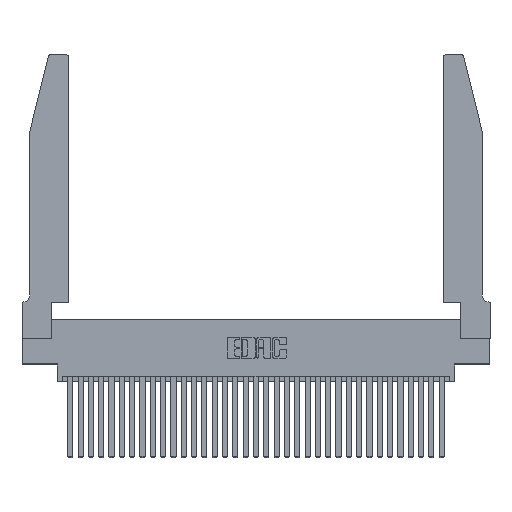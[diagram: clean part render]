
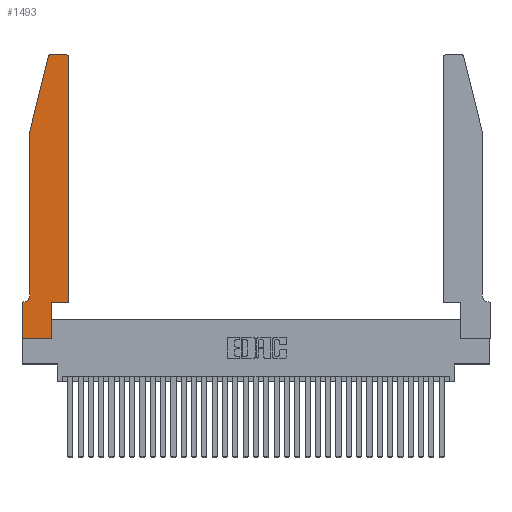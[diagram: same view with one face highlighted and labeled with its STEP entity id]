
A CAD part, top view. The second image highlights one B-rep face of the part: STEP entity #1493.
In plain terms, the highlighted planar face has unit normal (0, 0, 1).
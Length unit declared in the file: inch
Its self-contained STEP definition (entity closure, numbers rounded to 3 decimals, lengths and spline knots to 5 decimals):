
#58 = CARTESIAN_POINT ( 'NONE',  ( 0.284, 2.72, 0.37 ) ) ;
#142 = LINE ( 'NONE', #5960, #14579 ) ;
#613 = ORIENTED_EDGE ( 'NONE', *, *, #21931, .T. ) ;
#890 = DIRECTION ( 'NONE',  ( -1., 0., 0. ) ) ;
#907 = CARTESIAN_POINT ( 'NONE',  ( 0.0755, 2., 0.37 ) ) ;
#1493 = ADVANCED_FACE ( 'NONE', ( #13940 ), #15203, .T. ) ;
#1640 = VERTEX_POINT ( 'NONE', #9543 ) ;
#1760 = VECTOR ( 'NONE', #22726, 39.37008 ) ;
#1867 = VECTOR ( 'NONE', #25450, 39.37008 ) ;
#2013 = CIRCLE ( 'NONE', #11670, 0.03 ) ;
#2410 = VECTOR ( 'NONE', #11007, 39.37008 ) ;
#2797 = ORIENTED_EDGE ( 'NONE', *, *, #31492, .T. ) ;
#2894 = DIRECTION ( 'NONE',  ( 1., 0., 0. ) ) ;
#2965 = VECTOR ( 'NONE', #29072, 39.37008 ) ;
#4158 = LINE ( 'NONE', #26662, #2410 ) ;
#4244 = CARTESIAN_POINT ( 'NONE',  ( 0., 0., 0.37 ) ) ;
#5217 = EDGE_CURVE ( 'NONE', #7828, #17692, #23101, .T. ) ;
#5246 = VERTEX_POINT ( 'NONE', #30974 ) ;
#5944 = DIRECTION ( 'NONE',  ( 0., 1., 0. ) ) ;
#5960 = CARTESIAN_POINT ( 'NONE',  ( 0.0755, 2., 0.37 ) ) ;
#6598 = CARTESIAN_POINT ( 'NONE',  ( 0.25487, 2.72718, 0.37 ) ) ;
#6966 = CARTESIAN_POINT ( 'NONE',  ( 0.2605, 2.75, 0.37 ) ) ;
#7046 = DIRECTION ( 'NONE',  ( 0., 0., 1. ) ) ;
#7828 = VERTEX_POINT ( 'NONE', #10424 ) ;
#7961 = ORIENTED_EDGE ( 'NONE', *, *, #5217, .T. ) ;
#8370 = ORIENTED_EDGE ( 'NONE', *, *, #20316, .T. ) ;
#8818 = ORIENTED_EDGE ( 'NONE', *, *, #14589, .T. ) ;
#9064 = CARTESIAN_POINT ( 'NONE',  ( 0.0055, 0.35, 0.37 ) ) ;
#9543 = CARTESIAN_POINT ( 'NONE',  ( 0.0755, 0.42, 0.37 ) ) ;
#10069 = ORIENTED_EDGE ( 'NONE', *, *, #23558, .T. ) ;
#10424 = CARTESIAN_POINT ( 'NONE',  ( 0.4505, 0.35, 0.37 ) ) ;
#10915 = EDGE_CURVE ( 'NONE', #32493, #16985, #23509, .T. ) ;
#11007 = DIRECTION ( 'NONE',  ( -1., 0., 0. ) ) ;
#11014 = VERTEX_POINT ( 'NONE', #20634 ) ;
#11587 = CARTESIAN_POINT ( 'NONE',  ( 0., 0.35, 0.37 ) ) ;
#11670 = AXIS2_PLACEMENT_3D ( 'NONE', #22809, #7046, #25445 ) ;
#12025 = EDGE_CURVE ( 'NONE', #17823, #5246, #16896, .T. ) ;
#13385 = CARTESIAN_POINT ( 'NONE',  ( 0.4505, 0.35, 0.37 ) ) ;
#13393 = ORIENTED_EDGE ( 'NONE', *, *, #20196, .T. ) ;
#13940 = FACE_OUTER_BOUND ( 'NONE', #31649, .T. ) ;
#14579 = VECTOR ( 'NONE', #24386, 39.37008 ) ;
#14589 = EDGE_CURVE ( 'NONE', #17692, #17823, #2013, .T. ) ;
#14602 = ORIENTED_EDGE ( 'NONE', *, *, #12025, .T. ) ;
#14742 = DIRECTION ( 'NONE',  ( 1., 0., 0. ) ) ;
#14877 = CARTESIAN_POINT ( 'NONE',  ( 0.4505, 2.72, 0.37 ) ) ;
#14972 = DIRECTION ( 'NONE',  ( 0., 0., 1. ) ) ;
#15203 = PLANE ( 'NONE',  #16921 ) ;
#15237 = VECTOR ( 'NONE', #19773, 39.37008 ) ;
#15934 = LINE ( 'NONE', #24368, #29055 ) ;
#16250 = ORIENTED_EDGE ( 'NONE', *, *, #16742, .T. ) ;
#16601 = VECTOR ( 'NONE', #22777, 39.37008 ) ;
#16742 = EDGE_CURVE ( 'NONE', #23755, #1640, #142, .T. ) ;
#16896 = LINE ( 'NONE', #6966, #1760 ) ;
#16921 = AXIS2_PLACEMENT_3D ( 'NONE', #30317, #14972, #14742 ) ;
#16985 = VERTEX_POINT ( 'NONE', #4244 ) ;
#17044 = DIRECTION ( 'NONE',  ( 0., 0., -1. ) ) ;
#17692 = VERTEX_POINT ( 'NONE', #14877 ) ;
#17823 = VERTEX_POINT ( 'NONE', #25711 ) ;
#17949 = VERTEX_POINT ( 'NONE', #20928 ) ;
#18053 = LINE ( 'NONE', #13385, #2965 ) ;
#18458 = CIRCLE ( 'NONE', #32542, 0.07 ) ;
#18740 = ORIENTED_EDGE ( 'NONE', *, *, #10915, .T. ) ;
#18922 = DIRECTION ( 'NONE',  ( 0., 0., 1. ) ) ;
#18934 = LINE ( 'NONE', #33287, #25017 ) ;
#19221 = EDGE_CURVE ( 'NONE', #5246, #27080, #32523, .T. ) ;
#19773 = DIRECTION ( 'NONE',  ( 1., 0., 0. ) ) ;
#20196 = EDGE_CURVE ( 'NONE', #16985, #11014, #22161, .T. ) ;
#20232 = DIRECTION ( 'NONE',  ( -0.239, -0.971, 0. ) ) ;
#20316 = EDGE_CURVE ( 'NONE', #27080, #23755, #18934, .T. ) ;
#20634 = CARTESIAN_POINT ( 'NONE',  ( 0.2865, 0., 0.37 ) ) ;
#20928 = CARTESIAN_POINT ( 'NONE',  ( 0.2865, 0.35, 0.37 ) ) ;
#21931 = EDGE_CURVE ( 'NONE', #17949, #7828, #18053, .T. ) ;
#22152 = VERTEX_POINT ( 'NONE', #9064 ) ;
#22161 = LINE ( 'NONE', #27532, #15237 ) ;
#22726 = DIRECTION ( 'NONE',  ( -1., 0., 0. ) ) ;
#22777 = DIRECTION ( 'NONE',  ( 0., -1., 0. ) ) ;
#22809 = CARTESIAN_POINT ( 'NONE',  ( 0.4205, 2.72, 0.37 ) ) ;
#23101 = LINE ( 'NONE', #30746, #1867 ) ;
#23509 = LINE ( 'NONE', #25410, #16601 ) ;
#23558 = EDGE_CURVE ( 'NONE', #22152, #32493, #4158, .T. ) ;
#23755 = VERTEX_POINT ( 'NONE', #907 ) ;
#24368 = CARTESIAN_POINT ( 'NONE',  ( 0.2865, 0.35, 0.37 ) ) ;
#24386 = DIRECTION ( 'NONE',  ( 0., -1., 0. ) ) ;
#25017 = VECTOR ( 'NONE', #20232, 39.37008 ) ;
#25410 = CARTESIAN_POINT ( 'NONE',  ( 0., 0., 0.37 ) ) ;
#25445 = DIRECTION ( 'NONE',  ( 1., 0., 0. ) ) ;
#25450 = DIRECTION ( 'NONE',  ( 0., 1., 0. ) ) ;
#25711 = CARTESIAN_POINT ( 'NONE',  ( 0.4205, 2.75, 0.37 ) ) ;
#25962 = AXIS2_PLACEMENT_3D ( 'NONE', #58, #18922, #2894 ) ;
#26662 = CARTESIAN_POINT ( 'NONE',  ( 0.0755, 0.35, 0.37 ) ) ;
#27080 = VERTEX_POINT ( 'NONE', #6598 ) ;
#27279 = ORIENTED_EDGE ( 'NONE', *, *, #28049, .T. ) ;
#27532 = CARTESIAN_POINT ( 'NONE',  ( 0., 0., 0.37 ) ) ;
#28049 = EDGE_CURVE ( 'NONE', #11014, #17949, #15934, .T. ) ;
#28526 = ORIENTED_EDGE ( 'NONE', *, *, #19221, .T. ) ;
#29055 = VECTOR ( 'NONE', #5944, 39.37008 ) ;
#29072 = DIRECTION ( 'NONE',  ( 1., 0., 0. ) ) ;
#30317 = CARTESIAN_POINT ( 'NONE',  ( 0., 0.35, 0.37 ) ) ;
#30746 = CARTESIAN_POINT ( 'NONE',  ( 0.4505, 0.35, 0.37 ) ) ;
#30974 = CARTESIAN_POINT ( 'NONE',  ( 0.284, 2.75, 0.37 ) ) ;
#31492 = EDGE_CURVE ( 'NONE', #1640, #22152, #18458, .T. ) ;
#31649 = EDGE_LOOP ( 'NONE', ( #14602, #28526, #8370, #16250, #2797, #10069, #18740, #13393, #27279, #613, #7961, #8818 ) ) ;
#32493 = VERTEX_POINT ( 'NONE', #11587 ) ;
#32523 = CIRCLE ( 'NONE', #25962, 0.03 ) ;
#32542 = AXIS2_PLACEMENT_3D ( 'NONE', #32752, #17044, #890 ) ;
#32752 = CARTESIAN_POINT ( 'NONE',  ( 0.0055, 0.42, 0.37 ) ) ;
#33287 = CARTESIAN_POINT ( 'NONE',  ( 0.0755, 2., 0.37 ) ) ;
